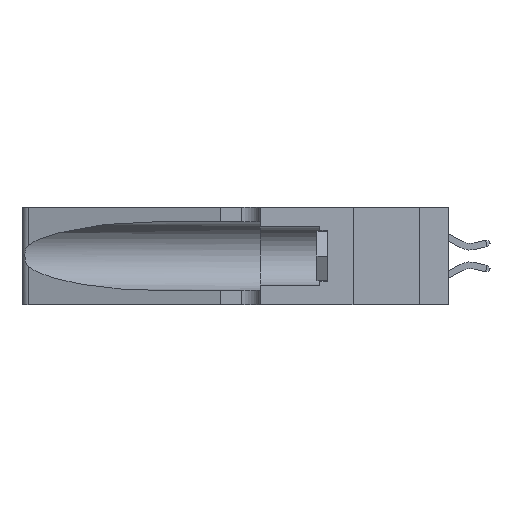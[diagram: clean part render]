
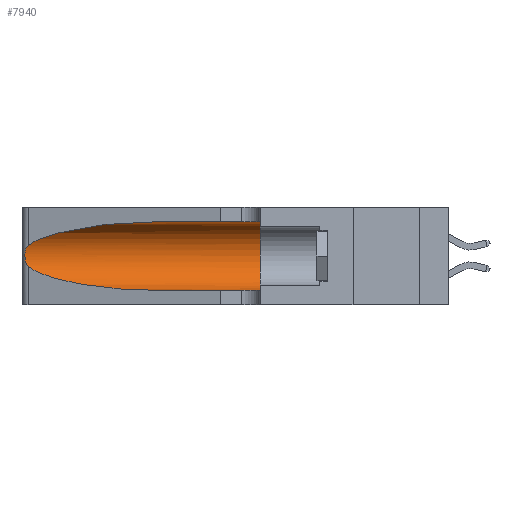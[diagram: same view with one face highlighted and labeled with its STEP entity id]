
A CAD part, left-side view. The second image highlights one B-rep face of the part: STEP entity #7940.
In plain terms, the highlighted cylindrical face has radius 3.308 mm (diameter 6.617 mm), a partial arc.
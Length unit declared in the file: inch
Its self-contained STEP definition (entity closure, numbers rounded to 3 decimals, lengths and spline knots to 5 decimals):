
#48 = AXIS2_PLACEMENT_3D ( 'NONE', #1483, #18719, #3711 ) ;
#1483 = CARTESIAN_POINT ( 'NONE',  ( 0.1305, 1.61858, 0.185 ) ) ;
#1647 = CARTESIAN_POINT ( 'NONE',  ( 0.26075, 1.23896, 0.178 ) ) ;
#1766 = ORIENTED_EDGE ( 'NONE', *, *, #25966, .T. ) ;
#1899 = CARTESIAN_POINT ( 'NONE',  ( 0.25487, 1.22718, 0.22369 ) ) ;
#2084 = VERTEX_POINT ( 'NONE', #1899 ) ;
#3630 = VECTOR ( 'NONE', #12111, 39.37008 ) ;
#3711 = DIRECTION ( 'NONE',  ( 0., 0., -1. ) ) ;
#3886 = CARTESIAN_POINT ( 'NONE',  ( 0.25856, 1.23593, 0.16098 ) ) ;
#4696 = CARTESIAN_POINT ( 'NONE',  ( 0.1305, 0.35, 0.185 ) ) ;
#5330 = VERTEX_POINT ( 'NONE', #26461 ) ;
#5773 = ORIENTED_EDGE ( 'NONE', *, *, #16026, .F. ) ;
#5898 = CARTESIAN_POINT ( 'NONE',  ( 0.18966, 0.96281, 0.31525 ) ) ;
#6052 =( BOUNDED_CURVE ( )  B_SPLINE_CURVE ( 3, ( #20850, #5898, #25031, #12448 ),
 .UNSPECIFIED., .F., .F. ) 
 B_SPLINE_CURVE_WITH_KNOTS ( ( 4, 4 ),
 ( 1.5708, 2.84003 ),
 .UNSPECIFIED. ) 
 CURVE ( )  GEOMETRIC_REPRESENTATION_ITEM ( )  RATIONAL_B_SPLINE_CURVE ( ( 1., 0.87, 0.87, 1. ) ) 
 REPRESENTATION_ITEM ( '' )  );
#6065 = CARTESIAN_POINT ( 'NONE',  ( 0.25639, 1.23186, 0.15144 ) ) ;
#6870 = DIRECTION ( 'NONE',  ( 0., 0., 1. ) ) ;
#7411 = ORIENTED_EDGE ( 'NONE', *, *, #10576, .F. ) ;
#7561 = AXIS2_PLACEMENT_3D ( 'NONE', #4696, #19672, #6870 ) ;
#7940 = ADVANCED_FACE ( 'NONE', ( #27147 ), #26501, .F. ) ;
#7945 = EDGE_CURVE ( 'NONE', #5330, #2084, #6052, .T. ) ;
#8174 = CARTESIAN_POINT ( 'NONE',  ( 0.25487, 1.22718, 0.22369 ) ) ;
#8268 = CARTESIAN_POINT ( 'NONE',  ( 0.25487, 1.22718, 0.14631 ) ) ;
#8950 = VERTEX_POINT ( 'NONE', #11274 ) ;
#9290 = CARTESIAN_POINT ( 'NONE',  ( 0.18966, 0.96281, 0.05475 ) ) ;
#9975 = DIRECTION ( 'NONE',  ( 0., -1., 0. ) ) ;
#10366 = CARTESIAN_POINT ( 'NONE',  ( 0.25639, 1.23184, 0.21858 ) ) ;
#10576 = EDGE_CURVE ( 'NONE', #5330, #15088, #24054, .T. ) ;
#11274 = CARTESIAN_POINT ( 'NONE',  ( 0.1305, 0.72297, 0.05475 ) ) ;
#12063 = ORIENTED_EDGE ( 'NONE', *, *, #18216, .T. ) ;
#12111 = DIRECTION ( 'NONE',  ( 0., -1., 0. ) ) ;
#12448 = CARTESIAN_POINT ( 'NONE',  ( 0.25487, 1.22718, 0.22369 ) ) ;
#12517 = CARTESIAN_POINT ( 'NONE',  ( 0.25854, 1.2359, 0.20912 ) ) ;
#12866 = VECTOR ( 'NONE', #9975, 39.37008 ) ;
#13041 = EDGE_LOOP ( 'NONE', ( #20617, #25336, #12063, #1766, #5773, #7411 ) ) ;
#14236 = CARTESIAN_POINT ( 'NONE',  ( 0.1305, 1.61858, 0.05475 ) ) ;
#14513 = VERTEX_POINT ( 'NONE', #20779 ) ;
#14640 = CARTESIAN_POINT ( 'NONE',  ( 0.26075, 1.23896, 0.19203 ) ) ;
#15088 = VERTEX_POINT ( 'NONE', #26682 ) ;
#15651 = CARTESIAN_POINT ( 'NONE',  ( 0.25487, 1.22718, 0.14631 ) ) ;
#16026 = EDGE_CURVE ( 'NONE', #15088, #14513, #27010, .T. ) ;
#16227 = CARTESIAN_POINT ( 'NONE',  ( 0.25487, 1.22718, 0.14631 ) ) ;
#16772 = CARTESIAN_POINT ( 'NONE',  ( 0.26017, 1.23833, 0.17102 ) ) ;
#16891 =( BOUNDED_CURVE ( )  B_SPLINE_CURVE ( 3, ( #15651, #21880, #9290, #24091 ),
 .UNSPECIFIED., .F., .F. ) 
 B_SPLINE_CURVE_WITH_KNOTS ( ( 4, 4 ),
 ( 3.44316, 4.71239 ),
 .UNSPECIFIED. ) 
 CURVE ( )  GEOMETRIC_REPRESENTATION_ITEM ( )  RATIONAL_B_SPLINE_CURVE ( ( 1., 0.87, 0.87, 1. ) ) 
 REPRESENTATION_ITEM ( '' )  );
#17863 = EDGE_CURVE ( 'NONE', #2084, #23909, #21766, .T. ) ;
#18216 = EDGE_CURVE ( 'NONE', #23909, #8950, #16891, .T. ) ;
#18415 = CARTESIAN_POINT ( 'NONE',  ( 0.1305, 1.61858, 0.31525 ) ) ;
#18719 = DIRECTION ( 'NONE',  ( 0., -1., 0. ) ) ;
#18882 = CARTESIAN_POINT ( 'NONE',  ( 0.25789, 1.23486, 0.15765 ) ) ;
#19672 = DIRECTION ( 'NONE',  ( 0., 1., 0. ) ) ;
#20617 = ORIENTED_EDGE ( 'NONE', *, *, #7945, .T. ) ;
#20733 = LINE ( 'NONE', #14236, #3630 ) ;
#20779 = CARTESIAN_POINT ( 'NONE',  ( 0.1305, 0.35, 0.05475 ) ) ;
#20850 = CARTESIAN_POINT ( 'NONE',  ( 0.1305, 0.72297, 0.31525 ) ) ;
#20920 = CARTESIAN_POINT ( 'NONE',  ( 0.25555, 1.22994, 0.2215 ) ) ;
#21009 = CARTESIAN_POINT ( 'NONE',  ( 0.25555, 1.22993, 0.14849 ) ) ;
#21766 = B_SPLINE_CURVE_WITH_KNOTS ( 'NONE', 3,
 ( #8174, #20920, #10366, #25108, #12517, #27211, #14640, #1647, #16772, #3886, #18882, #6065, #21009, #8268 ),
 .UNSPECIFIED., .F., .F.,
 ( 4, 2, 2, 2, 2, 2, 4 ),
 ( 0., 0.00027, 0.00053, 0.00107, 0.0016, 0.00187, 0.00214 ),
 .UNSPECIFIED. ) ;
#21880 = CARTESIAN_POINT ( 'NONE',  ( 0.2373, 1.15595, 0.08982 ) ) ;
#23909 = VERTEX_POINT ( 'NONE', #16227 ) ;
#24054 = LINE ( 'NONE', #18415, #12866 ) ;
#24091 = CARTESIAN_POINT ( 'NONE',  ( 0.1305, 0.72297, 0.05475 ) ) ;
#25031 = CARTESIAN_POINT ( 'NONE',  ( 0.2373, 1.15595, 0.28018 ) ) ;
#25108 = CARTESIAN_POINT ( 'NONE',  ( 0.25787, 1.23484, 0.2124 ) ) ;
#25336 = ORIENTED_EDGE ( 'NONE', *, *, #17863, .T. ) ;
#25966 = EDGE_CURVE ( 'NONE', #8950, #14513, #20733, .T. ) ;
#26461 = CARTESIAN_POINT ( 'NONE',  ( 0.1305, 0.72297, 0.31525 ) ) ;
#26501 = CYLINDRICAL_SURFACE ( 'NONE', #48, 0.13025 ) ;
#26682 = CARTESIAN_POINT ( 'NONE',  ( 0.1305, 0.35, 0.31525 ) ) ;
#27010 = CIRCLE ( 'NONE', #7561, 0.13025 ) ;
#27147 = FACE_OUTER_BOUND ( 'NONE', #13041, .T. ) ;
#27211 = CARTESIAN_POINT ( 'NONE',  ( 0.26018, 1.23835, 0.19895 ) ) ;
